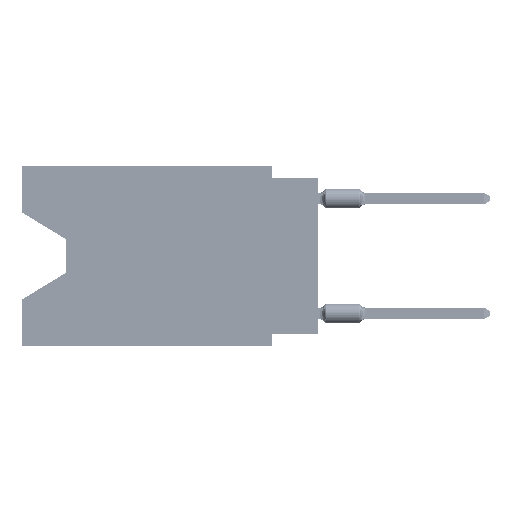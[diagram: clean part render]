
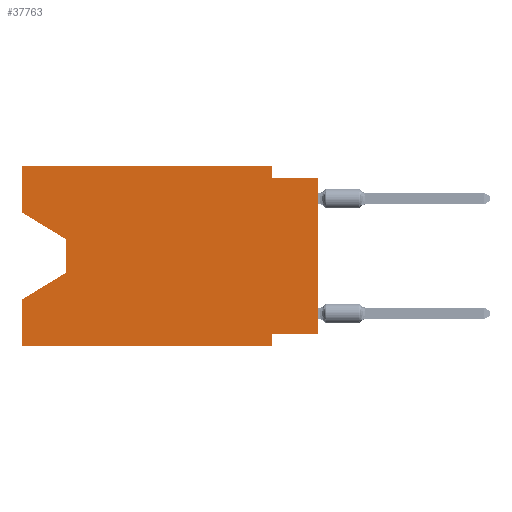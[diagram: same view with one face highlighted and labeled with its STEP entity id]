
A CAD part, left-side view. The second image highlights one B-rep face of the part: STEP entity #37763.
In plain terms, the highlighted planar face has unit normal (-1, 0, 0).
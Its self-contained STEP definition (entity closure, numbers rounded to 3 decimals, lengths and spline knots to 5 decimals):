
#159 = VERTEX_POINT ( 'NONE', #3852 ) ;
#1684 = ORIENTED_EDGE ( 'NONE', *, *, #47524, .F. ) ;
#2092 = VERTEX_POINT ( 'NONE', #17695 ) ;
#2333 = AXIS2_PLACEMENT_3D ( 'NONE', #15776, #2530, #54608 ) ;
#2418 = CARTESIAN_POINT ( 'NONE',  ( 0., 0., -0.025 ) ) ;
#2530 = DIRECTION ( 'NONE',  ( 1., 0., 0. ) ) ;
#2701 = VECTOR ( 'NONE', #15279, 39.37008 ) ;
#3852 = CARTESIAN_POINT ( 'NONE',  ( 0., 0.645, 0. ) ) ;
#7485 = LINE ( 'NONE', #35714, #52432 ) ;
#8365 = DIRECTION ( 'NONE',  ( 0., -1., 0. ) ) ;
#8498 = DIRECTION ( 'NONE',  ( 0., -0.855, -0.519 ) ) ;
#8632 = CARTESIAN_POINT ( 'NONE',  ( 0., 0.1, 0. ) ) ;
#9384 = ORIENTED_EDGE ( 'NONE', *, *, #27857, .F. ) ;
#9706 = CARTESIAN_POINT ( 'NONE',  ( 0., 0.645, -0.39 ) ) ;
#11252 = LINE ( 'NONE', #65947, #38633 ) ;
#12031 = EDGE_CURVE ( 'NONE', #52506, #2092, #30738, .T. ) ;
#12487 = DIRECTION ( 'NONE',  ( 0., 0., -1. ) ) ;
#12698 = FACE_OUTER_BOUND ( 'NONE', #29631, .T. ) ;
#12914 = CARTESIAN_POINT ( 'NONE',  ( 0., 0.645, 0. ) ) ;
#14036 = EDGE_CURVE ( 'NONE', #81928, #72620, #87092, .T. ) ;
#14660 = ORIENTED_EDGE ( 'NONE', *, *, #77838, .T. ) ;
#15279 = DIRECTION ( 'NONE',  ( 0., -1., 0. ) ) ;
#15574 = LINE ( 'NONE', #37164, #29372 ) ;
#15776 = CARTESIAN_POINT ( 'NONE',  ( 0., 0.645, 0. ) ) ;
#16691 = VECTOR ( 'NONE', #30561, 39.37008 ) ;
#17695 = CARTESIAN_POINT ( 'NONE',  ( 0., 0.1, -0.025 ) ) ;
#20128 = VECTOR ( 'NONE', #72955, 39.37008 ) ;
#20555 = CARTESIAN_POINT ( 'NONE',  ( 0., 0.55, -0.158 ) ) ;
#22949 = EDGE_CURVE ( 'NONE', #56110, #159, #15574, .T. ) ;
#23081 = VERTEX_POINT ( 'NONE', #57901 ) ;
#23507 = CARTESIAN_POINT ( 'NONE',  ( 0., 0., 0. ) ) ;
#23861 = ORIENTED_EDGE ( 'NONE', *, *, #42435, .T. ) ;
#25929 = LINE ( 'NONE', #52870, #71829 ) ;
#27435 = VERTEX_POINT ( 'NONE', #2418 ) ;
#27857 = EDGE_CURVE ( 'NONE', #62081, #23081, #39425, .T. ) ;
#29372 = VECTOR ( 'NONE', #77344, 39.37008 ) ;
#29631 = EDGE_LOOP ( 'NONE', ( #74289, #23861, #75214, #61734, #41866, #9384, #1684, #14660, #45029, #32794, #62525, #57302 ) ) ;
#30561 = DIRECTION ( 'NONE',  ( 0., 0., 1. ) ) ;
#30738 = LINE ( 'NONE', #48867, #46845 ) ;
#32147 = EDGE_CURVE ( 'NONE', #2092, #27435, #7485, .T. ) ;
#32794 = ORIENTED_EDGE ( 'NONE', *, *, #12031, .F. ) ;
#33080 = LINE ( 'NONE', #86095, #79063 ) ;
#33527 = VERTEX_POINT ( 'NONE', #35298 ) ;
#33770 = CARTESIAN_POINT ( 'NONE',  ( 0., 0., -0.365 ) ) ;
#35298 = CARTESIAN_POINT ( 'NONE',  ( 0., 0.55, -0.232 ) ) ;
#35714 = CARTESIAN_POINT ( 'NONE',  ( 0., 0., -0.025 ) ) ;
#35847 = CARTESIAN_POINT ( 'NONE',  ( 0., 0.645, -0.10025 ) ) ;
#35998 = LINE ( 'NONE', #75732, #2701 ) ;
#37164 = CARTESIAN_POINT ( 'NONE',  ( 0., 0.645, 0. ) ) ;
#37763 = ADVANCED_FACE ( 'NONE', ( #12698 ), #40064, .F. ) ;
#38488 = LINE ( 'NONE', #23507, #16691 ) ;
#38633 = VECTOR ( 'NONE', #80831, 39.37008 ) ;
#39425 = LINE ( 'NONE', #52251, #52203 ) ;
#39480 = VECTOR ( 'NONE', #8498, 39.37008 ) ;
#39523 = DIRECTION ( 'NONE',  ( 0., 1., 0. ) ) ;
#40064 = PLANE ( 'NONE',  #2333 ) ;
#41273 = CARTESIAN_POINT ( 'NONE',  ( 0., 0., -0.365 ) ) ;
#41866 = ORIENTED_EDGE ( 'NONE', *, *, #65090, .T. ) ;
#42435 = EDGE_CURVE ( 'NONE', #77032, #33527, #25929, .T. ) ;
#42686 = DIRECTION ( 'NONE',  ( 0., 0., -1. ) ) ;
#43050 = VERTEX_POINT ( 'NONE', #41273 ) ;
#44194 = EDGE_CURVE ( 'NONE', #159, #52506, #33080, .T. ) ;
#45029 = ORIENTED_EDGE ( 'NONE', *, *, #32147, .F. ) ;
#46761 = DIRECTION ( 'NONE',  ( 0., -1., 0. ) ) ;
#46845 = VECTOR ( 'NONE', #42686, 39.37008 ) ;
#47410 = CARTESIAN_POINT ( 'NONE',  ( 0., 0.1, -0.365 ) ) ;
#47524 = EDGE_CURVE ( 'NONE', #43050, #62081, #60695, .T. ) ;
#48867 = CARTESIAN_POINT ( 'NONE',  ( 0., 0.1, 0. ) ) ;
#52203 = VECTOR ( 'NONE', #12487, 39.37008 ) ;
#52251 = CARTESIAN_POINT ( 'NONE',  ( 0., 0.1, -0.39 ) ) ;
#52432 = VECTOR ( 'NONE', #8365, 39.37008 ) ;
#52506 = VERTEX_POINT ( 'NONE', #8632 ) ;
#52870 = CARTESIAN_POINT ( 'NONE',  ( 0., 0.55, -0.158 ) ) ;
#53532 = LINE ( 'NONE', #35847, #39480 ) ;
#53968 = VECTOR ( 'NONE', #39523, 39.37008 ) ;
#54608 = DIRECTION ( 'NONE',  ( 0., 0., -1. ) ) ;
#56110 = VERTEX_POINT ( 'NONE', #78973 ) ;
#57302 = ORIENTED_EDGE ( 'NONE', *, *, #22949, .F. ) ;
#57901 = CARTESIAN_POINT ( 'NONE',  ( 0., 0.1, -0.39 ) ) ;
#60695 = LINE ( 'NONE', #33770, #53968 ) ;
#61734 = ORIENTED_EDGE ( 'NONE', *, *, #14036, .F. ) ;
#62081 = VERTEX_POINT ( 'NONE', #47410 ) ;
#62525 = ORIENTED_EDGE ( 'NONE', *, *, #44194, .F. ) ;
#65090 = EDGE_CURVE ( 'NONE', #81928, #23081, #35998, .T. ) ;
#65947 = CARTESIAN_POINT ( 'NONE',  ( 0., 0.55, -0.232 ) ) ;
#70974 = EDGE_CURVE ( 'NONE', #33527, #72620, #11252, .T. ) ;
#71829 = VECTOR ( 'NONE', #72730, 39.37008 ) ;
#72620 = VERTEX_POINT ( 'NONE', #76905 ) ;
#72730 = DIRECTION ( 'NONE',  ( 0., 0., -1. ) ) ;
#72955 = DIRECTION ( 'NONE',  ( 0., 0., 1. ) ) ;
#74289 = ORIENTED_EDGE ( 'NONE', *, *, #80201, .T. ) ;
#75214 = ORIENTED_EDGE ( 'NONE', *, *, #70974, .T. ) ;
#75732 = CARTESIAN_POINT ( 'NONE',  ( 0., 0.645, -0.39 ) ) ;
#76905 = CARTESIAN_POINT ( 'NONE',  ( 0., 0.645, -0.28975 ) ) ;
#77032 = VERTEX_POINT ( 'NONE', #20555 ) ;
#77344 = DIRECTION ( 'NONE',  ( 0., 0., 1. ) ) ;
#77838 = EDGE_CURVE ( 'NONE', #43050, #27435, #38488, .T. ) ;
#78973 = CARTESIAN_POINT ( 'NONE',  ( 0., 0.645, -0.10025 ) ) ;
#79063 = VECTOR ( 'NONE', #46761, 39.37008 ) ;
#80201 = EDGE_CURVE ( 'NONE', #56110, #77032, #53532, .T. ) ;
#80831 = DIRECTION ( 'NONE',  ( 0., 0.855, -0.519 ) ) ;
#81928 = VERTEX_POINT ( 'NONE', #9706 ) ;
#86095 = CARTESIAN_POINT ( 'NONE',  ( 0., 0.645, 0. ) ) ;
#87092 = LINE ( 'NONE', #12914, #20128 ) ;
